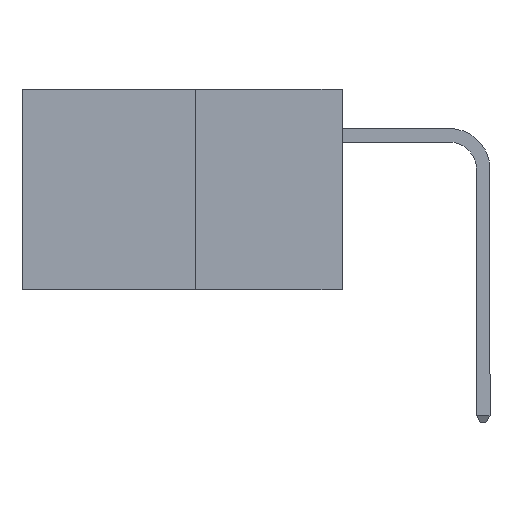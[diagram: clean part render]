
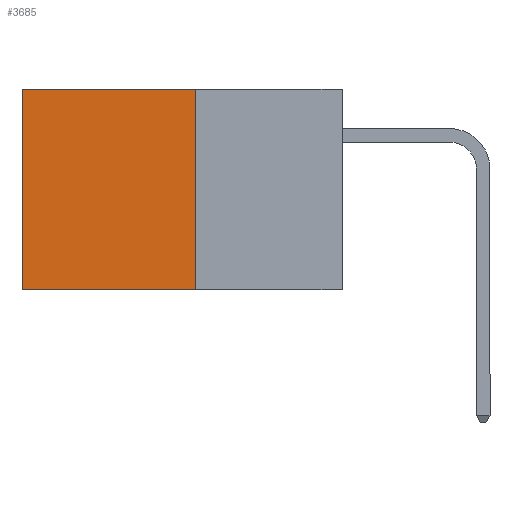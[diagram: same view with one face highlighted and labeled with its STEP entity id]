
A CAD part, left-side view. The second image highlights one B-rep face of the part: STEP entity #3685.
In plain terms, the highlighted planar face has unit normal (-1, 0, 0).
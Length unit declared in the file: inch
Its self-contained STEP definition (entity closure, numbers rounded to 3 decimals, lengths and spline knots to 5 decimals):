
#155 = LINE ( 'NONE', #6282, #3327 ) ;
#163 = VECTOR ( 'NONE', #1185, 39.37008 ) ;
#398 = ORIENTED_EDGE ( 'NONE', *, *, #6072, .T. ) ;
#1124 = EDGE_CURVE ( 'NONE', #7718, #5816, #155, .T. ) ;
#1185 = DIRECTION ( 'NONE',  ( 0., 0., -1. ) ) ;
#1280 = DIRECTION ( 'NONE',  ( 0., 1., 0. ) ) ;
#1347 = AXIS2_PLACEMENT_3D ( 'NONE', #4868, #4877, #7801 ) ;
#1651 = DIRECTION ( 'NONE',  ( 0., 1., 0. ) ) ;
#1685 = VERTEX_POINT ( 'NONE', #2308 ) ;
#1699 = EDGE_LOOP ( 'NONE', ( #398, #3764, #2296, #5533 ) ) ;
#1837 = CARTESIAN_POINT ( 'NONE',  ( 0.277, 0.59, -0.37 ) ) ;
#2004 = EDGE_CURVE ( 'NONE', #1685, #3636, #2039, .T. ) ;
#2039 = LINE ( 'NONE', #3165, #5101 ) ;
#2296 = ORIENTED_EDGE ( 'NONE', *, *, #6158, .F. ) ;
#2308 = CARTESIAN_POINT ( 'NONE',  ( 0.277, 0.27, 0. ) ) ;
#3165 = CARTESIAN_POINT ( 'NONE',  ( 0.277, 0.27, 0. ) ) ;
#3192 = FACE_OUTER_BOUND ( 'NONE', #1699, .T. ) ;
#3327 = VECTOR ( 'NONE', #1651, 39.37008 ) ;
#3522 = LINE ( 'NONE', #1837, #163 ) ;
#3636 = VERTEX_POINT ( 'NONE', #4598 ) ;
#3685 = ADVANCED_FACE ( 'NONE', ( #3192 ), #5099, .F. ) ;
#3764 = ORIENTED_EDGE ( 'NONE', *, *, #1124, .F. ) ;
#4386 = VECTOR ( 'NONE', #7378, 39.37008 ) ;
#4598 = CARTESIAN_POINT ( 'NONE',  ( 0.277, 0.59, 0. ) ) ;
#4765 = CARTESIAN_POINT ( 'NONE',  ( 0.277, 0.27, -0.37 ) ) ;
#4868 = CARTESIAN_POINT ( 'NONE',  ( 0.277, 0.27, -0.37 ) ) ;
#4877 = DIRECTION ( 'NONE',  ( 1., 0., 0. ) ) ;
#4941 = CARTESIAN_POINT ( 'NONE',  ( 0.277, 0.59, -0.37 ) ) ;
#5099 = PLANE ( 'NONE',  #1347 ) ;
#5101 = VECTOR ( 'NONE', #1280, 39.37008 ) ;
#5533 = ORIENTED_EDGE ( 'NONE', *, *, #2004, .T. ) ;
#5568 = CARTESIAN_POINT ( 'NONE',  ( 0.277, 0.27, -0.37 ) ) ;
#5816 = VERTEX_POINT ( 'NONE', #4941 ) ;
#5957 = LINE ( 'NONE', #5568, #4386 ) ;
#6072 = EDGE_CURVE ( 'NONE', #3636, #5816, #3522, .T. ) ;
#6158 = EDGE_CURVE ( 'NONE', #1685, #7718, #5957, .T. ) ;
#6282 = CARTESIAN_POINT ( 'NONE',  ( 0.277, 0.27, -0.37 ) ) ;
#7378 = DIRECTION ( 'NONE',  ( 0., 0., -1. ) ) ;
#7718 = VERTEX_POINT ( 'NONE', #4765 ) ;
#7801 = DIRECTION ( 'NONE',  ( 0., 0., -1. ) ) ;
